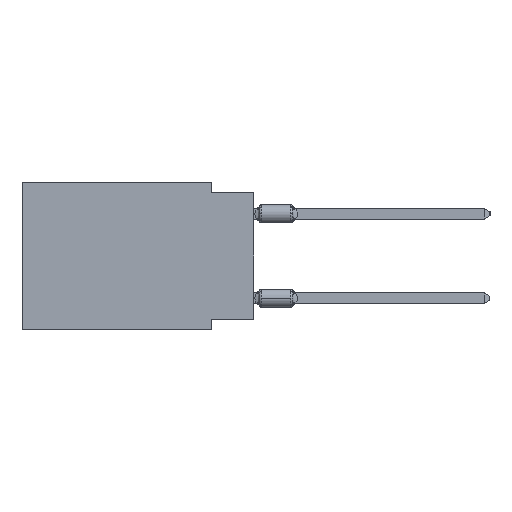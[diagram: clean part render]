
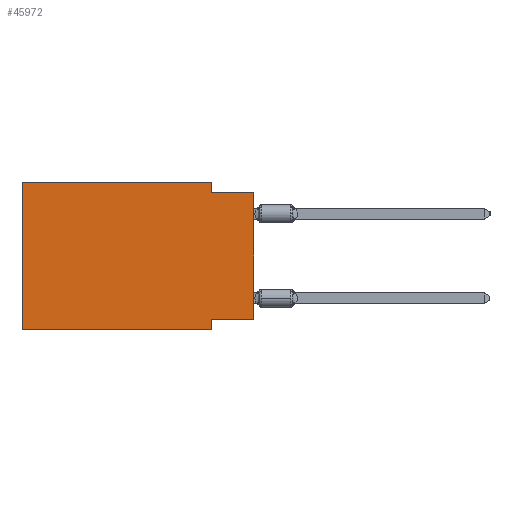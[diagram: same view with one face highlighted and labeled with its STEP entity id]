
A CAD part, left-side view. The second image highlights one B-rep face of the part: STEP entity #45972.
In plain terms, the highlighted planar face has unit normal (-1, 0, 0).
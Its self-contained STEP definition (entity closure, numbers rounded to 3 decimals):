
#235 = CARTESIAN_POINT ( 'NONE',  ( 0., 2.54, -8.89 ) ) ;
#767 = DIRECTION ( 'NONE',  ( 0., 0., -1. ) ) ;
#1739 = LINE ( 'NONE', #18124, #9248 ) ;
#1851 = EDGE_CURVE ( 'NONE', #35878, #41116, #48236, .T. ) ;
#2761 = VERTEX_POINT ( 'NONE', #26456 ) ;
#2935 = CARTESIAN_POINT ( 'NONE',  ( 0., 13.97, 0. ) ) ;
#4666 = CARTESIAN_POINT ( 'NONE',  ( 0., 0., -8.255 ) ) ;
#6061 = EDGE_CURVE ( 'NONE', #33692, #37255, #46136, .T. ) ;
#7031 = EDGE_LOOP ( 'NONE', ( #42345, #22285, #11600, #22953, #12829, #51068, #50521, #36816 ) ) ;
#7382 = CARTESIAN_POINT ( 'NONE',  ( 0., 13.97, -8.89 ) ) ;
#7694 = DIRECTION ( 'NONE',  ( 0., -1., 0. ) ) ;
#7709 = DIRECTION ( 'NONE',  ( 0., 0., 1. ) ) ;
#8229 = DIRECTION ( 'NONE',  ( 0., 0., -1. ) ) ;
#9248 = VECTOR ( 'NONE', #21884, 1000. ) ;
#11413 = LINE ( 'NONE', #7382, #17879 ) ;
#11600 = ORIENTED_EDGE ( 'NONE', *, *, #33607, .F. ) ;
#12829 = ORIENTED_EDGE ( 'NONE', *, *, #52237, .F. ) ;
#13304 = PLANE ( 'NONE',  #52452 ) ;
#14621 = VERTEX_POINT ( 'NONE', #26557 ) ;
#15677 = EDGE_CURVE ( 'NONE', #46363, #33692, #20687, .T. ) ;
#15755 = CARTESIAN_POINT ( 'NONE',  ( 0., 13.97, 0. ) ) ;
#16007 = DIRECTION ( 'NONE',  ( 0., 0., -1. ) ) ;
#17879 = VECTOR ( 'NONE', #35575, 1000. ) ;
#18124 = CARTESIAN_POINT ( 'NONE',  ( 0., 0., 0. ) ) ;
#19556 = LINE ( 'NONE', #23578, #35064 ) ;
#20138 = CARTESIAN_POINT ( 'NONE',  ( 0., 0., -0.635 ) ) ;
#20687 = LINE ( 'NONE', #28212, #20786 ) ;
#20786 = VECTOR ( 'NONE', #24199, 1000. ) ;
#21884 = DIRECTION ( 'NONE',  ( 0., 0., 1. ) ) ;
#22285 = ORIENTED_EDGE ( 'NONE', *, *, #22911, .F. ) ;
#22911 = EDGE_CURVE ( 'NONE', #30131, #14621, #28186, .T. ) ;
#22953 = ORIENTED_EDGE ( 'NONE', *, *, #1851, .F. ) ;
#23578 = CARTESIAN_POINT ( 'NONE',  ( 0., 13.97, 0. ) ) ;
#24199 = DIRECTION ( 'NONE',  ( 0., 1., 0. ) ) ;
#26356 = VECTOR ( 'NONE', #16007, 1000. ) ;
#26456 = CARTESIAN_POINT ( 'NONE',  ( 0., 13.97, -8.89 ) ) ;
#26557 = CARTESIAN_POINT ( 'NONE',  ( 0., 0., -0.635 ) ) ;
#27926 = DIRECTION ( 'NONE',  ( 0., -1., 0. ) ) ;
#28186 = LINE ( 'NONE', #20138, #45078 ) ;
#28212 = CARTESIAN_POINT ( 'NONE',  ( 0., 0., -8.255 ) ) ;
#29424 = DIRECTION ( 'NONE',  ( 1., 0., 0. ) ) ;
#30131 = VERTEX_POINT ( 'NONE', #38378 ) ;
#33433 = CARTESIAN_POINT ( 'NONE',  ( 0., 2.54, -8.255 ) ) ;
#33607 = EDGE_CURVE ( 'NONE', #41116, #30131, #36402, .T. ) ;
#33692 = VERTEX_POINT ( 'NONE', #33433 ) ;
#35064 = VECTOR ( 'NONE', #7709, 1000. ) ;
#35242 = CARTESIAN_POINT ( 'NONE',  ( 0., 2.54, -8.89 ) ) ;
#35575 = DIRECTION ( 'NONE',  ( 0., -1., 0. ) ) ;
#35878 = VERTEX_POINT ( 'NONE', #2935 ) ;
#36402 = LINE ( 'NONE', #52776, #26356 ) ;
#36816 = ORIENTED_EDGE ( 'NONE', *, *, #15677, .F. ) ;
#37255 = VERTEX_POINT ( 'NONE', #35242 ) ;
#37983 = CARTESIAN_POINT ( 'NONE',  ( 0., 13.97, 0. ) ) ;
#38360 = VECTOR ( 'NONE', #7694, 1000. ) ;
#38378 = CARTESIAN_POINT ( 'NONE',  ( 0., 2.54, -0.635 ) ) ;
#40143 = CARTESIAN_POINT ( 'NONE',  ( 0., 2.54, 0. ) ) ;
#41049 = EDGE_CURVE ( 'NONE', #2761, #37255, #11413, .T. ) ;
#41116 = VERTEX_POINT ( 'NONE', #40143 ) ;
#42345 = ORIENTED_EDGE ( 'NONE', *, *, #47065, .T. ) ;
#45078 = VECTOR ( 'NONE', #27926, 1000. ) ;
#45972 = ADVANCED_FACE ( 'NONE', ( #46063 ), #13304, .F. ) ;
#46063 = FACE_OUTER_BOUND ( 'NONE', #7031, .T. ) ;
#46136 = LINE ( 'NONE', #235, #51877 ) ;
#46363 = VERTEX_POINT ( 'NONE', #4666 ) ;
#47065 = EDGE_CURVE ( 'NONE', #46363, #14621, #1739, .T. ) ;
#48236 = LINE ( 'NONE', #15755, #38360 ) ;
#50521 = ORIENTED_EDGE ( 'NONE', *, *, #6061, .F. ) ;
#51068 = ORIENTED_EDGE ( 'NONE', *, *, #41049, .T. ) ;
#51877 = VECTOR ( 'NONE', #767, 1000. ) ;
#52237 = EDGE_CURVE ( 'NONE', #2761, #35878, #19556, .T. ) ;
#52452 = AXIS2_PLACEMENT_3D ( 'NONE', #37983, #29424, #8229 ) ;
#52776 = CARTESIAN_POINT ( 'NONE',  ( 0., 2.54, 0. ) ) ;
